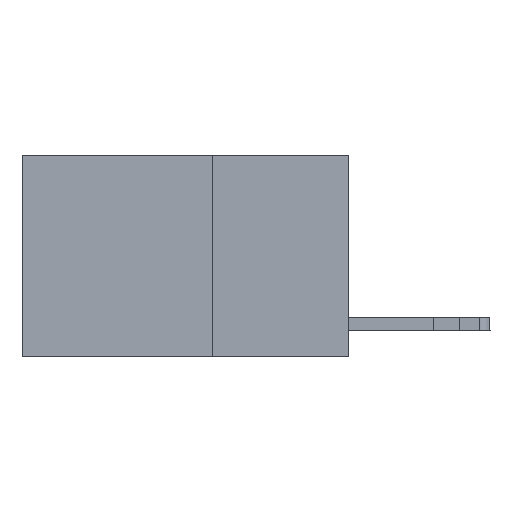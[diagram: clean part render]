
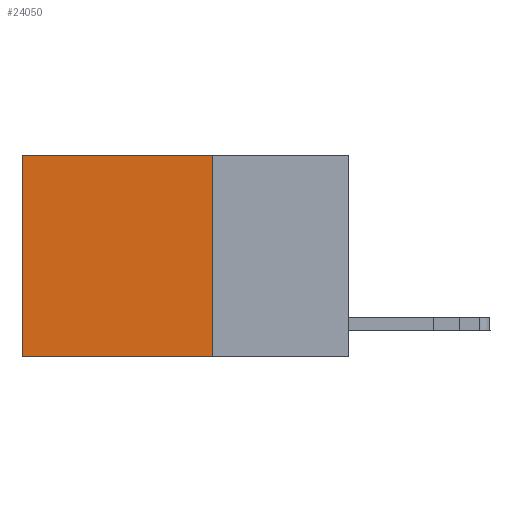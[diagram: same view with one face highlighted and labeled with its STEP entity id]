
A CAD part, left-side view. The second image highlights one B-rep face of the part: STEP entity #24050.
In plain terms, the highlighted planar face has unit normal (-1, 0, 0).
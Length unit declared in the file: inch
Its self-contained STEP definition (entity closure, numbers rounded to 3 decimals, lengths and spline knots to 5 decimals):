
#12 = CARTESIAN_POINT ( 'NONE',  ( 0.2625, 0.6, 0. ) ) ;
#1025 = EDGE_CURVE ( 'NONE', #17327, #6915, #1558, .T. ) ;
#1340 = LINE ( 'NONE', #18042, #15604 ) ;
#1558 = LINE ( 'NONE', #1681, #7521 ) ;
#1603 = CARTESIAN_POINT ( 'NONE',  ( 0.2625, 0.25, 0. ) ) ;
#1642 = CARTESIAN_POINT ( 'NONE',  ( 0.2625, 0.6, -0.37 ) ) ;
#1681 = CARTESIAN_POINT ( 'NONE',  ( 0.2625, 0.25, 0. ) ) ;
#1904 = ORIENTED_EDGE ( 'NONE', *, *, #5544, .F. ) ;
#3123 = ORIENTED_EDGE ( 'NONE', *, *, #1025, .F. ) ;
#4809 = CARTESIAN_POINT ( 'NONE',  ( 0.2625, 0.25, -0.37 ) ) ;
#5544 = EDGE_CURVE ( 'NONE', #6915, #13566, #14884, .T. ) ;
#6915 = VERTEX_POINT ( 'NONE', #23404 ) ;
#7521 = VECTOR ( 'NONE', #26323, 39.37008 ) ;
#7631 = DIRECTION ( 'NONE',  ( 0., 0., -1. ) ) ;
#10031 = PLANE ( 'NONE',  #12339 ) ;
#10071 = VECTOR ( 'NONE', #7631, 39.37008 ) ;
#12212 = VERTEX_POINT ( 'NONE', #12 ) ;
#12339 = AXIS2_PLACEMENT_3D ( 'NONE', #1603, #20756, #24721 ) ;
#13566 = VERTEX_POINT ( 'NONE', #1642 ) ;
#14646 = EDGE_LOOP ( 'NONE', ( #20861, #1904, #3123, #16243 ) ) ;
#14884 = LINE ( 'NONE', #4809, #21002 ) ;
#15604 = VECTOR ( 'NONE', #19823, 39.37008 ) ;
#16207 = CARTESIAN_POINT ( 'NONE',  ( 0.2625, 0.6, 0. ) ) ;
#16243 = ORIENTED_EDGE ( 'NONE', *, *, #16900, .T. ) ;
#16900 = EDGE_CURVE ( 'NONE', #17327, #12212, #1340, .T. ) ;
#17327 = VERTEX_POINT ( 'NONE', #18000 ) ;
#18000 = CARTESIAN_POINT ( 'NONE',  ( 0.2625, 0.25, 0. ) ) ;
#18042 = CARTESIAN_POINT ( 'NONE',  ( 0.2625, 0.25, 0. ) ) ;
#19823 = DIRECTION ( 'NONE',  ( 0., 1., 0. ) ) ;
#20398 = LINE ( 'NONE', #16207, #10071 ) ;
#20756 = DIRECTION ( 'NONE',  ( 1., 0., 0. ) ) ;
#20861 = ORIENTED_EDGE ( 'NONE', *, *, #26111, .T. ) ;
#21002 = VECTOR ( 'NONE', #25509, 39.37008 ) ;
#23404 = CARTESIAN_POINT ( 'NONE',  ( 0.2625, 0.25, -0.37 ) ) ;
#24050 = ADVANCED_FACE ( 'NONE', ( #26647 ), #10031, .F. ) ;
#24721 = DIRECTION ( 'NONE',  ( 0., 0., -1. ) ) ;
#25509 = DIRECTION ( 'NONE',  ( 0., 1., 0. ) ) ;
#26111 = EDGE_CURVE ( 'NONE', #12212, #13566, #20398, .T. ) ;
#26323 = DIRECTION ( 'NONE',  ( 0., 0., -1. ) ) ;
#26647 = FACE_OUTER_BOUND ( 'NONE', #14646, .T. ) ;
